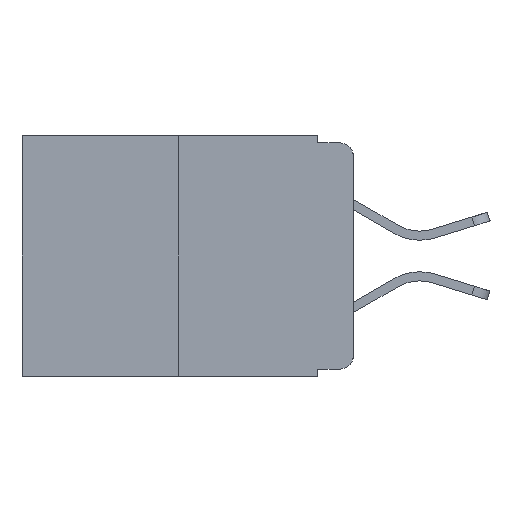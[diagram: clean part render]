
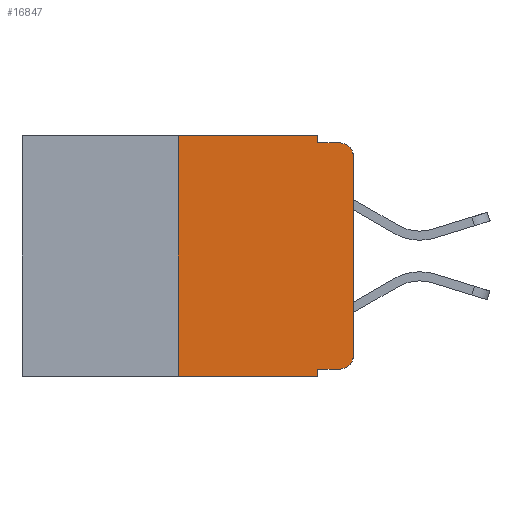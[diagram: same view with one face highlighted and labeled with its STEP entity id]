
A CAD part, left-side view. The second image highlights one B-rep face of the part: STEP entity #16847.
In plain terms, the highlighted planar face has unit normal (-1, 0, 0).
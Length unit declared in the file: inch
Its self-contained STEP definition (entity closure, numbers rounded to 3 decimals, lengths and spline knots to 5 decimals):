
#21 = CARTESIAN_POINT ( 'NONE',  ( 0., 0.051, 0. ) ) ;
#194 = CARTESIAN_POINT ( 'NONE',  ( 0., 0.02, -0.01 ) ) ;
#206 = VERTEX_POINT ( 'NONE', #10998 ) ;
#854 = VERTEX_POINT ( 'NONE', #10584 ) ;
#1286 = ORIENTED_EDGE ( 'NONE', *, *, #6840, .F. ) ;
#1648 = DIRECTION ( 'NONE',  ( 0., 0., -1. ) ) ;
#1787 = DIRECTION ( 'NONE',  ( 0., 0., -1. ) ) ;
#1901 = CARTESIAN_POINT ( 'NONE',  ( 0., 0.25, -0.343 ) ) ;
#2097 = DIRECTION ( 'NONE',  ( -1., 0., 0. ) ) ;
#2223 = LINE ( 'NONE', #14099, #9423 ) ;
#2435 = EDGE_CURVE ( 'NONE', #8891, #3787, #9184, .T. ) ;
#2458 = FACE_OUTER_BOUND ( 'NONE', #5983, .T. ) ;
#2546 = VERTEX_POINT ( 'NONE', #9797 ) ;
#2621 = ORIENTED_EDGE ( 'NONE', *, *, #6573, .T. ) ;
#2769 = DIRECTION ( 'NONE',  ( 0., 0., 1. ) ) ;
#3533 = CARTESIAN_POINT ( 'NONE',  ( 0., 0.02, -0.03 ) ) ;
#3622 = LINE ( 'NONE', #14846, #11261 ) ;
#3687 = LINE ( 'NONE', #5083, #11816 ) ;
#3787 = VERTEX_POINT ( 'NONE', #12021 ) ;
#3987 = CIRCLE ( 'NONE', #8164, 0.02 ) ;
#4188 = ORIENTED_EDGE ( 'NONE', *, *, #5600, .F. ) ;
#4807 = LINE ( 'NONE', #21, #8650 ) ;
#4831 = VECTOR ( 'NONE', #18593, 39.37008 ) ;
#4914 = EDGE_CURVE ( 'NONE', #15354, #854, #3622, .T. ) ;
#4936 = CARTESIAN_POINT ( 'NONE',  ( 0., 0.051, -0.333 ) ) ;
#5083 = CARTESIAN_POINT ( 'NONE',  ( 0., 0.051, -0.01 ) ) ;
#5157 = DIRECTION ( 'NONE',  ( 0., 0., -1. ) ) ;
#5600 = EDGE_CURVE ( 'NONE', #9410, #206, #7159, .T. ) ;
#5711 = ORIENTED_EDGE ( 'NONE', *, *, #2435, .T. ) ;
#5983 = EDGE_LOOP ( 'NONE', ( #2621, #11308, #11803, #20646, #4188, #8542, #17502, #1286, #5711, #10057 ) ) ;
#6228 = CARTESIAN_POINT ( 'NONE',  ( 0., 0.25, 0. ) ) ;
#6498 = CARTESIAN_POINT ( 'NONE',  ( 0., 0.473, 0. ) ) ;
#6573 = EDGE_CURVE ( 'NONE', #2546, #14521, #2223, .T. ) ;
#6840 = EDGE_CURVE ( 'NONE', #8891, #854, #4807, .T. ) ;
#6887 = DIRECTION ( 'NONE',  ( 0., -1., 0. ) ) ;
#7159 = LINE ( 'NONE', #14887, #7677 ) ;
#7677 = VECTOR ( 'NONE', #6887, 39.37008 ) ;
#8164 = AXIS2_PLACEMENT_3D ( 'NONE', #3533, #14791, #5157 ) ;
#8439 = DIRECTION ( 'NONE',  ( 0., -1., 0. ) ) ;
#8542 = ORIENTED_EDGE ( 'NONE', *, *, #19774, .F. ) ;
#8650 = VECTOR ( 'NONE', #1787, 39.37008 ) ;
#8767 = EDGE_CURVE ( 'NONE', #14521, #18814, #3987, .T. ) ;
#8891 = VERTEX_POINT ( 'NONE', #13434 ) ;
#9184 = LINE ( 'NONE', #4936, #4831 ) ;
#9410 = VERTEX_POINT ( 'NONE', #19657 ) ;
#9423 = VECTOR ( 'NONE', #2769, 39.37008 ) ;
#9525 = AXIS2_PLACEMENT_3D ( 'NONE', #6498, #11478, #1648 ) ;
#9797 = CARTESIAN_POINT ( 'NONE',  ( 0., 0., -0.313 ) ) ;
#10057 = ORIENTED_EDGE ( 'NONE', *, *, #18862, .T. ) ;
#10584 = CARTESIAN_POINT ( 'NONE',  ( 0., 0.051, -0.343 ) ) ;
#10605 = VERTEX_POINT ( 'NONE', #15261 ) ;
#10998 = CARTESIAN_POINT ( 'NONE',  ( 0., 0.051, 0. ) ) ;
#11027 = AXIS2_PLACEMENT_3D ( 'NONE', #11886, #2097, #13490 ) ;
#11261 = VECTOR ( 'NONE', #8439, 39.37008 ) ;
#11308 = ORIENTED_EDGE ( 'NONE', *, *, #8767, .T. ) ;
#11478 = DIRECTION ( 'NONE',  ( 1., 0., 0. ) ) ;
#11627 = LINE ( 'NONE', #16872, #20462 ) ;
#11803 = ORIENTED_EDGE ( 'NONE', *, *, #18732, .F. ) ;
#11816 = VECTOR ( 'NONE', #16317, 39.37008 ) ;
#11886 = CARTESIAN_POINT ( 'NONE',  ( 0., 0.02, -0.313 ) ) ;
#12021 = CARTESIAN_POINT ( 'NONE',  ( 0., 0.02, -0.333 ) ) ;
#12091 = DIRECTION ( 'NONE',  ( 0., 0., -1. ) ) ;
#13434 = CARTESIAN_POINT ( 'NONE',  ( 0., 0.051, -0.333 ) ) ;
#13490 = DIRECTION ( 'NONE',  ( 0., 0., -1. ) ) ;
#14037 = CIRCLE ( 'NONE', #11027, 0.02 ) ;
#14099 = CARTESIAN_POINT ( 'NONE',  ( 0., 0., 0. ) ) ;
#14521 = VERTEX_POINT ( 'NONE', #15615 ) ;
#14791 = DIRECTION ( 'NONE',  ( -1., 0., 0. ) ) ;
#14846 = CARTESIAN_POINT ( 'NONE',  ( 0., 0.473, -0.343 ) ) ;
#14887 = CARTESIAN_POINT ( 'NONE',  ( 0., 0.473, 0. ) ) ;
#15261 = CARTESIAN_POINT ( 'NONE',  ( 0., 0.051, -0.01 ) ) ;
#15354 = VERTEX_POINT ( 'NONE', #1901 ) ;
#15615 = CARTESIAN_POINT ( 'NONE',  ( 0., 0., -0.03 ) ) ;
#16317 = DIRECTION ( 'NONE',  ( 0., -1., 0. ) ) ;
#16726 = LINE ( 'NONE', #6228, #20869 ) ;
#16847 = ADVANCED_FACE ( 'NONE', ( #2458 ), #19335, .F. ) ;
#16872 = CARTESIAN_POINT ( 'NONE',  ( 0., 0.051, 0. ) ) ;
#17502 = ORIENTED_EDGE ( 'NONE', *, *, #4914, .T. ) ;
#17695 = EDGE_CURVE ( 'NONE', #206, #10605, #11627, .T. ) ;
#18593 = DIRECTION ( 'NONE',  ( 0., -1., 0. ) ) ;
#18732 = EDGE_CURVE ( 'NONE', #10605, #18814, #3687, .T. ) ;
#18814 = VERTEX_POINT ( 'NONE', #194 ) ;
#18862 = EDGE_CURVE ( 'NONE', #3787, #2546, #14037, .T. ) ;
#19020 = DIRECTION ( 'NONE',  ( 0., 0., 1. ) ) ;
#19335 = PLANE ( 'NONE',  #9525 ) ;
#19657 = CARTESIAN_POINT ( 'NONE',  ( 0., 0.25, 0. ) ) ;
#19774 = EDGE_CURVE ( 'NONE', #15354, #9410, #16726, .T. ) ;
#20462 = VECTOR ( 'NONE', #12091, 39.37008 ) ;
#20646 = ORIENTED_EDGE ( 'NONE', *, *, #17695, .F. ) ;
#20869 = VECTOR ( 'NONE', #19020, 39.37008 ) ;
